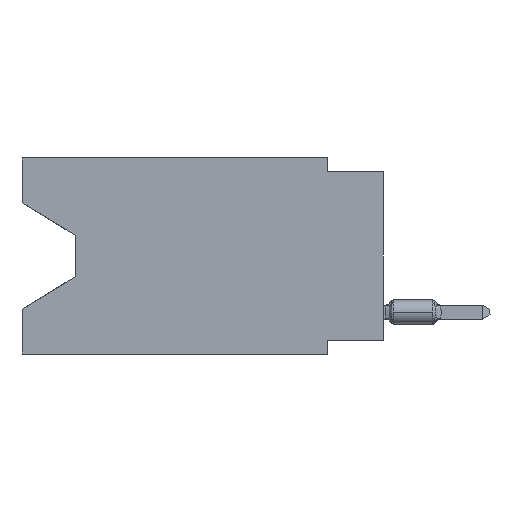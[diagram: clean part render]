
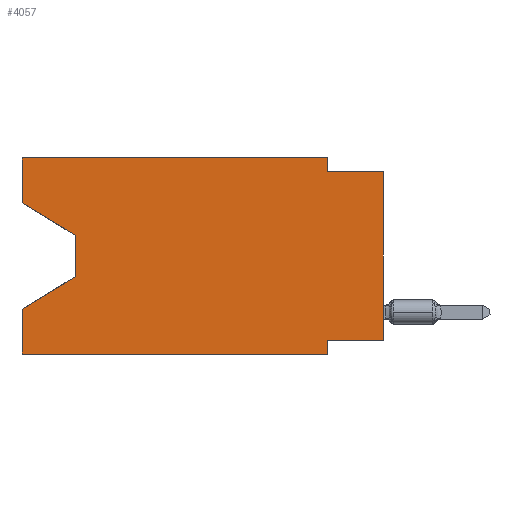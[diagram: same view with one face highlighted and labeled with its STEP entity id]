
A CAD part, left-side view. The second image highlights one B-rep face of the part: STEP entity #4057.
In plain terms, the highlighted planar face has unit normal (-1, 0, 0).
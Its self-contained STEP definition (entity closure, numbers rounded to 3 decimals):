
#584 = VECTOR ( 'NONE', #24533, 1000. ) ;
#1312 = DIRECTION ( 'NONE',  ( 0., 0.855, -0.519 ) ) ;
#1464 = CARTESIAN_POINT ( 'NONE',  ( 0., 16.383, 0. ) ) ;
#1758 = VECTOR ( 'NONE', #9305, 1000. ) ;
#2332 = EDGE_CURVE ( 'NONE', #3257, #23635, #20014, .T. ) ;
#2412 = CARTESIAN_POINT ( 'NONE',  ( 0., 0., 0. ) ) ;
#2470 = VECTOR ( 'NONE', #1312, 1000. ) ;
#2573 = VERTEX_POINT ( 'NONE', #18586 ) ;
#2574 = LINE ( 'NONE', #11823, #15573 ) ;
#3257 = VERTEX_POINT ( 'NONE', #16242 ) ;
#3275 = VERTEX_POINT ( 'NONE', #6471 ) ;
#3288 = DIRECTION ( 'NONE',  ( 1., 0., 0. ) ) ;
#3332 = EDGE_CURVE ( 'NONE', #13206, #23567, #15055, .T. ) ;
#3465 = DIRECTION ( 'NONE',  ( 0., 0., -1. ) ) ;
#4057 = ADVANCED_FACE ( 'NONE', ( #24659 ), #16764, .F. ) ;
#4370 = DIRECTION ( 'NONE',  ( 0., -1., 0. ) ) ;
#5182 = LINE ( 'NONE', #1464, #1758 ) ;
#5206 = LINE ( 'NONE', #10496, #584 ) ;
#5241 = CARTESIAN_POINT ( 'NONE',  ( 0., 13.97, -3.505 ) ) ;
#5355 = AXIS2_PLACEMENT_3D ( 'NONE', #14595, #3288, #24409 ) ;
#6228 = EDGE_CURVE ( 'NONE', #10695, #23635, #25242, .T. ) ;
#6329 = CARTESIAN_POINT ( 'NONE',  ( 0., 2.54, -8.89 ) ) ;
#6471 = CARTESIAN_POINT ( 'NONE',  ( 0., 13.97, -3.505 ) ) ;
#6520 = CARTESIAN_POINT ( 'NONE',  ( 0., 16.383, -8.89 ) ) ;
#6528 = EDGE_CURVE ( 'NONE', #3257, #13230, #24685, .T. ) ;
#7059 = EDGE_CURVE ( 'NONE', #3275, #13206, #24834, .T. ) ;
#7105 = CARTESIAN_POINT ( 'NONE',  ( 0., 16.383, -2.038 ) ) ;
#7431 = ORIENTED_EDGE ( 'NONE', *, *, #3332, .T. ) ;
#7577 = CARTESIAN_POINT ( 'NONE',  ( 0., 0., -0.635 ) ) ;
#8121 = LINE ( 'NONE', #21916, #17135 ) ;
#8495 = ORIENTED_EDGE ( 'NONE', *, *, #18540, .F. ) ;
#9218 = ORIENTED_EDGE ( 'NONE', *, *, #7059, .T. ) ;
#9305 = DIRECTION ( 'NONE',  ( 0., 0., 1. ) ) ;
#9599 = VERTEX_POINT ( 'NONE', #7105 ) ;
#9778 = ORIENTED_EDGE ( 'NONE', *, *, #22255, .T. ) ;
#9822 = VECTOR ( 'NONE', #16156, 1000. ) ;
#10072 = LINE ( 'NONE', #11132, #13734 ) ;
#10496 = CARTESIAN_POINT ( 'NONE',  ( 0., 16.383, 0. ) ) ;
#10514 = ORIENTED_EDGE ( 'NONE', *, *, #18696, .F. ) ;
#10695 = VERTEX_POINT ( 'NONE', #22352 ) ;
#11000 = ORIENTED_EDGE ( 'NONE', *, *, #2332, .T. ) ;
#11015 = VECTOR ( 'NONE', #15404, 1000. ) ;
#11132 = CARTESIAN_POINT ( 'NONE',  ( 0., 2.54, 0. ) ) ;
#11438 = LINE ( 'NONE', #17354, #24996 ) ;
#11823 = CARTESIAN_POINT ( 'NONE',  ( 0., 16.383, -8.89 ) ) ;
#11900 = VERTEX_POINT ( 'NONE', #14611 ) ;
#11989 = DIRECTION ( 'NONE',  ( 0., -1., 0. ) ) ;
#12825 = EDGE_CURVE ( 'NONE', #13379, #11900, #2574, .T. ) ;
#13206 = VERTEX_POINT ( 'NONE', #17845 ) ;
#13230 = VERTEX_POINT ( 'NONE', #17726 ) ;
#13379 = VERTEX_POINT ( 'NONE', #6520 ) ;
#13734 = VECTOR ( 'NONE', #25063, 1000. ) ;
#14170 = DIRECTION ( 'NONE',  ( 0., 0., -1. ) ) ;
#14595 = CARTESIAN_POINT ( 'NONE',  ( 0., 16.383, 0. ) ) ;
#14611 = CARTESIAN_POINT ( 'NONE',  ( 0., 2.54, -8.89 ) ) ;
#14619 = CARTESIAN_POINT ( 'NONE',  ( 0., 0., -8.255 ) ) ;
#14987 = CARTESIAN_POINT ( 'NONE',  ( 0., 16.383, -6.852 ) ) ;
#15055 = LINE ( 'NONE', #15197, #2470 ) ;
#15080 = EDGE_CURVE ( 'NONE', #13379, #23567, #5182, .T. ) ;
#15197 = CARTESIAN_POINT ( 'NONE',  ( 0., 13.97, -5.385 ) ) ;
#15404 = DIRECTION ( 'NONE',  ( 0., -1., 0. ) ) ;
#15408 = DIRECTION ( 'NONE',  ( 0., -0.855, -0.519 ) ) ;
#15510 = VECTOR ( 'NONE', #22483, 1000. ) ;
#15573 = VECTOR ( 'NONE', #4370, 1000. ) ;
#15691 = ORIENTED_EDGE ( 'NONE', *, *, #15080, .F. ) ;
#16156 = DIRECTION ( 'NONE',  ( 0., 0., 1. ) ) ;
#16242 = CARTESIAN_POINT ( 'NONE',  ( 0., 0., -8.255 ) ) ;
#16764 = PLANE ( 'NONE',  #5355 ) ;
#16835 = CARTESIAN_POINT ( 'NONE',  ( 0., 16.383, 0. ) ) ;
#17135 = VECTOR ( 'NONE', #11989, 1000. ) ;
#17354 = CARTESIAN_POINT ( 'NONE',  ( 0., 16.383, -2.038 ) ) ;
#17726 = CARTESIAN_POINT ( 'NONE',  ( 0., 2.54, -8.255 ) ) ;
#17845 = CARTESIAN_POINT ( 'NONE',  ( 0., 13.97, -5.385 ) ) ;
#18007 = ORIENTED_EDGE ( 'NONE', *, *, #21966, .F. ) ;
#18540 = EDGE_CURVE ( 'NONE', #9599, #22035, #5206, .T. ) ;
#18586 = CARTESIAN_POINT ( 'NONE',  ( 0., 2.54, 0. ) ) ;
#18609 = CARTESIAN_POINT ( 'NONE',  ( 0., 0., -0.635 ) ) ;
#18696 = EDGE_CURVE ( 'NONE', #2573, #10695, #10072, .T. ) ;
#20014 = LINE ( 'NONE', #2412, #9822 ) ;
#20090 = VECTOR ( 'NONE', #3465, 1000. ) ;
#20353 = ORIENTED_EDGE ( 'NONE', *, *, #21880, .F. ) ;
#21376 = ORIENTED_EDGE ( 'NONE', *, *, #6228, .F. ) ;
#21880 = EDGE_CURVE ( 'NONE', #22035, #2573, #8121, .T. ) ;
#21916 = CARTESIAN_POINT ( 'NONE',  ( 0., 16.383, 0. ) ) ;
#21966 = EDGE_CURVE ( 'NONE', #13230, #11900, #23973, .T. ) ;
#22035 = VERTEX_POINT ( 'NONE', #16835 ) ;
#22255 = EDGE_CURVE ( 'NONE', #9599, #3275, #11438, .T. ) ;
#22352 = CARTESIAN_POINT ( 'NONE',  ( 0., 2.54, -0.635 ) ) ;
#22365 = ORIENTED_EDGE ( 'NONE', *, *, #6528, .F. ) ;
#22483 = DIRECTION ( 'NONE',  ( 0., 1., 0. ) ) ;
#22755 = ORIENTED_EDGE ( 'NONE', *, *, #12825, .T. ) ;
#23329 = EDGE_LOOP ( 'NONE', ( #9778, #9218, #7431, #15691, #22755, #18007, #22365, #11000, #21376, #10514, #20353, #8495 ) ) ;
#23567 = VERTEX_POINT ( 'NONE', #14987 ) ;
#23635 = VERTEX_POINT ( 'NONE', #18609 ) ;
#23742 = VECTOR ( 'NONE', #14170, 1000. ) ;
#23973 = LINE ( 'NONE', #6329, #23742 ) ;
#24409 = DIRECTION ( 'NONE',  ( 0., 0., -1. ) ) ;
#24533 = DIRECTION ( 'NONE',  ( 0., 0., 1. ) ) ;
#24659 = FACE_OUTER_BOUND ( 'NONE', #23329, .T. ) ;
#24685 = LINE ( 'NONE', #14619, #15510 ) ;
#24834 = LINE ( 'NONE', #5241, #20090 ) ;
#24996 = VECTOR ( 'NONE', #15408, 1000. ) ;
#25063 = DIRECTION ( 'NONE',  ( 0., 0., -1. ) ) ;
#25242 = LINE ( 'NONE', #7577, #11015 ) ;
